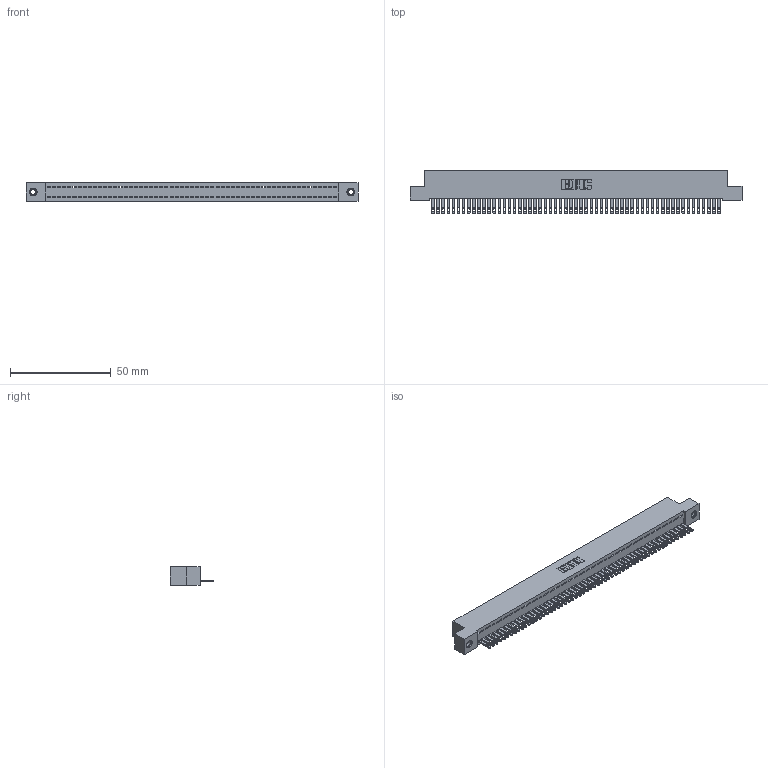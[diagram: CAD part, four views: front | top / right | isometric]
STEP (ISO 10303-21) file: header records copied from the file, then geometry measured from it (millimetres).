
FILE_DESCRIPTION (( 'STEP AP203' ), '1' );
FILE_NAME ('342-057-500-107.STEP', '2018-08-13T04:16:42', ( '' ), ( '' ), 'SwSTEP 2.0', 'SolidWorks 2016', '' );
FILE_SCHEMA (( 'CONFIG_CONTROL_DESIGN' ));
Length unit declared in the file: inch
Products named in the file (4): 345-250-001_345-250-005-103; 342-057-500-107; 342 Part_TI; 345-292-001_345-293-100
Assembly tree (60 placements, depth 2):
  342-057-500-107
    342 Part_TI
    345-292-001_345-293-100  x57
    345-250-001_345-250-005-103  x2
Bounding box: 165.1 x 21.85 x 9.4 mm (x, y, z)
Volume: 14553.8 mm3; surface area: 21796.1 mm2
Topology: 60 solids, 60 shells, 3248 faces, 10011 edges, 6666 vertices
Faces by surface type: plane 2150, cylinder 1082, cone 12, torus 4
Entity records: 33890 total; most frequent: CARTESIAN_POINT 5824, ORIENTED_EDGE 5810, DIRECTION 4917, EDGE_CURVE 2905, LINE 2753, VECTOR 2753, VERTEX_POINT 1932, AXIS2_PLACEMENT_3D 1082
